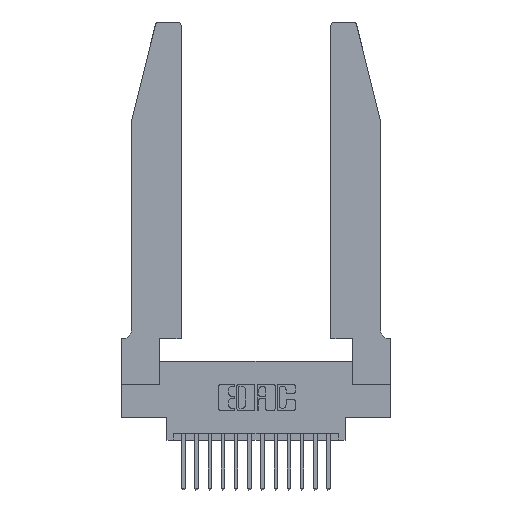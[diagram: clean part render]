
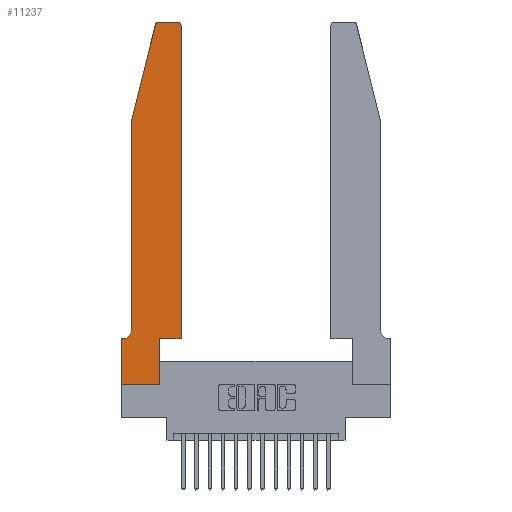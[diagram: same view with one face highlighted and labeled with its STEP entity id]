
A CAD part, top view. The second image highlights one B-rep face of the part: STEP entity #11237.
In plain terms, the highlighted planar face has unit normal (0, 0, 1).
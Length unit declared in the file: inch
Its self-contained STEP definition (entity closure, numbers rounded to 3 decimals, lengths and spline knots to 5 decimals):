
#123 = EDGE_CURVE ( 'NONE', #6997, #11160, #590, .T. ) ;
#590 = LINE ( 'NONE', #8348, #17667 ) ;
#595 = VECTOR ( 'NONE', #2272, 39.37008 ) ;
#698 = CARTESIAN_POINT ( 'NONE',  ( 0.2865, 0.35, 0.37 ) ) ;
#736 = ORIENTED_EDGE ( 'NONE', *, *, #9424, .T. ) ;
#827 = FACE_OUTER_BOUND ( 'NONE', #8961, .T. ) ;
#870 = LINE ( 'NONE', #10296, #5294 ) ;
#1381 = CARTESIAN_POINT ( 'NONE',  ( 0.2865, 0.35, 0.37 ) ) ;
#1463 = CARTESIAN_POINT ( 'NONE',  ( 0., 0., 0.37 ) ) ;
#1509 = CARTESIAN_POINT ( 'NONE',  ( 0., 0.35, 0.37 ) ) ;
#1594 = VERTEX_POINT ( 'NONE', #3056 ) ;
#1901 = CARTESIAN_POINT ( 'NONE',  ( 0.0755, 0.42, 0.37 ) ) ;
#1957 = ORIENTED_EDGE ( 'NONE', *, *, #18181, .T. ) ;
#2272 = DIRECTION ( 'NONE',  ( 1., 0., 0. ) ) ;
#2346 = EDGE_CURVE ( 'NONE', #17652, #11881, #870, .T. ) ;
#2435 = DIRECTION ( 'NONE',  ( 0., 0., 1. ) ) ;
#2855 = CARTESIAN_POINT ( 'NONE',  ( 0.25487, 2.72718, 0.37 ) ) ;
#2873 = ORIENTED_EDGE ( 'NONE', *, *, #4333, .T. ) ;
#2969 = ORIENTED_EDGE ( 'NONE', *, *, #4697, .T. ) ;
#3056 = CARTESIAN_POINT ( 'NONE',  ( 0.0755, 2., 0.37 ) ) ;
#3243 = CARTESIAN_POINT ( 'NONE',  ( 0.0755, 2., 0.37 ) ) ;
#3302 = LINE ( 'NONE', #13647, #17789 ) ;
#3532 = VERTEX_POINT ( 'NONE', #17469 ) ;
#4275 = CARTESIAN_POINT ( 'NONE',  ( 0.0755, 0.35, 0.37 ) ) ;
#4320 = DIRECTION ( 'NONE',  ( 1., 0., 0. ) ) ;
#4333 = EDGE_CURVE ( 'NONE', #5399, #3532, #4551, .T. ) ;
#4551 = LINE ( 'NONE', #9466, #595 ) ;
#4697 = EDGE_CURVE ( 'NONE', #1594, #5414, #14672, .T. ) ;
#5294 = VECTOR ( 'NONE', #10854, 39.37008 ) ;
#5344 = ORIENTED_EDGE ( 'NONE', *, *, #13227, .T. ) ;
#5399 = VERTEX_POINT ( 'NONE', #11874 ) ;
#5414 = VERTEX_POINT ( 'NONE', #1901 ) ;
#5489 = CARTESIAN_POINT ( 'NONE',  ( 0.284, 2.75, 0.37 ) ) ;
#6190 = DIRECTION ( 'NONE',  ( 0., -1., 0. ) ) ;
#6212 = EDGE_CURVE ( 'NONE', #11881, #6997, #9613, .T. ) ;
#6568 = DIRECTION ( 'NONE',  ( 0., 1., 0. ) ) ;
#6668 = ORIENTED_EDGE ( 'NONE', *, *, #6212, .T. ) ;
#6692 = VECTOR ( 'NONE', #8637, 39.37008 ) ;
#6775 = EDGE_CURVE ( 'NONE', #3532, #16432, #8300, .T. ) ;
#6997 = VERTEX_POINT ( 'NONE', #16781 ) ;
#7239 = CARTESIAN_POINT ( 'NONE',  ( 0.4505, 0.35, 0.37 ) ) ;
#7266 = VERTEX_POINT ( 'NONE', #8049 ) ;
#7330 = DIRECTION ( 'NONE',  ( -1., 0., 0. ) ) ;
#7344 = LINE ( 'NONE', #7239, #9823 ) ;
#7353 = AXIS2_PLACEMENT_3D ( 'NONE', #7497, #17211, #8926 ) ;
#7425 = ORIENTED_EDGE ( 'NONE', *, *, #2346, .T. ) ;
#7467 = ORIENTED_EDGE ( 'NONE', *, *, #123, .T. ) ;
#7497 = CARTESIAN_POINT ( 'NONE',  ( 0.284, 2.72, 0.37 ) ) ;
#7501 = ORIENTED_EDGE ( 'NONE', *, *, #6775, .T. ) ;
#7906 = DIRECTION ( 'NONE',  ( 0., 0., -1. ) ) ;
#8049 = CARTESIAN_POINT ( 'NONE',  ( 0.0055, 0.35, 0.37 ) ) ;
#8300 = LINE ( 'NONE', #698, #16101 ) ;
#8348 = CARTESIAN_POINT ( 'NONE',  ( 0.2605, 2.75, 0.37 ) ) ;
#8485 = DIRECTION ( 'NONE',  ( 0., 0., 1. ) ) ;
#8622 = AXIS2_PLACEMENT_3D ( 'NONE', #11003, #2435, #12408 ) ;
#8637 = DIRECTION ( 'NONE',  ( -1., 0., 0. ) ) ;
#8710 = EDGE_CURVE ( 'NONE', #7266, #10005, #10415, .T. ) ;
#8803 = DIRECTION ( 'NONE',  ( 0., -1., 0. ) ) ;
#8926 = DIRECTION ( 'NONE',  ( 1., 0., 0. ) ) ;
#8961 = EDGE_LOOP ( 'NONE', ( #7467, #11362, #18249, #2969, #1957, #15100, #5344, #2873, #7501, #736, #7425, #6668 ) ) ;
#9424 = EDGE_CURVE ( 'NONE', #16432, #17652, #7344, .T. ) ;
#9466 = CARTESIAN_POINT ( 'NONE',  ( 0., 0., 0.37 ) ) ;
#9613 = CIRCLE ( 'NONE', #8622, 0.03 ) ;
#9806 = PLANE ( 'NONE',  #17016 ) ;
#9823 = VECTOR ( 'NONE', #4320, 39.37008 ) ;
#9967 = CIRCLE ( 'NONE', #17928, 0.07 ) ;
#10005 = VERTEX_POINT ( 'NONE', #1509 ) ;
#10115 = VECTOR ( 'NONE', #6190, 39.37008 ) ;
#10296 = CARTESIAN_POINT ( 'NONE',  ( 0.4505, 0.35, 0.37 ) ) ;
#10415 = LINE ( 'NONE', #4275, #6692 ) ;
#10854 = DIRECTION ( 'NONE',  ( 0., 1., 0. ) ) ;
#11003 = CARTESIAN_POINT ( 'NONE',  ( 0.4205, 2.72, 0.37 ) ) ;
#11160 = VERTEX_POINT ( 'NONE', #5489 ) ;
#11237 = ADVANCED_FACE ( 'NONE', ( #827 ), #9806, .T. ) ;
#11362 = ORIENTED_EDGE ( 'NONE', *, *, #15876, .T. ) ;
#11874 = CARTESIAN_POINT ( 'NONE',  ( 0., 0., 0.37 ) ) ;
#11881 = VERTEX_POINT ( 'NONE', #16748 ) ;
#12408 = DIRECTION ( 'NONE',  ( 1., 0., 0. ) ) ;
#13227 = EDGE_CURVE ( 'NONE', #10005, #5399, #17639, .T. ) ;
#13647 = CARTESIAN_POINT ( 'NONE',  ( 0.0755, 2., 0.37 ) ) ;
#13977 = VECTOR ( 'NONE', #8803, 39.37008 ) ;
#14672 = LINE ( 'NONE', #3243, #10115 ) ;
#15063 = DIRECTION ( 'NONE',  ( -0.239, -0.971, 0. ) ) ;
#15100 = ORIENTED_EDGE ( 'NONE', *, *, #8710, .T. ) ;
#15824 = VERTEX_POINT ( 'NONE', #2855 ) ;
#15876 = EDGE_CURVE ( 'NONE', #11160, #15824, #16113, .T. ) ;
#16101 = VECTOR ( 'NONE', #6568, 39.37008 ) ;
#16113 = CIRCLE ( 'NONE', #7353, 0.03 ) ;
#16211 = CARTESIAN_POINT ( 'NONE',  ( 0.0055, 0.42, 0.37 ) ) ;
#16432 = VERTEX_POINT ( 'NONE', #1381 ) ;
#16686 = EDGE_CURVE ( 'NONE', #15824, #1594, #3302, .T. ) ;
#16748 = CARTESIAN_POINT ( 'NONE',  ( 0.4505, 2.72, 0.37 ) ) ;
#16773 = CARTESIAN_POINT ( 'NONE',  ( 0., 0.35, 0.37 ) ) ;
#16781 = CARTESIAN_POINT ( 'NONE',  ( 0.4205, 2.75, 0.37 ) ) ;
#17016 = AXIS2_PLACEMENT_3D ( 'NONE', #16773, #8485, #18147 ) ;
#17207 = CARTESIAN_POINT ( 'NONE',  ( 0.4505, 0.35, 0.37 ) ) ;
#17211 = DIRECTION ( 'NONE',  ( 0., 0., 1. ) ) ;
#17469 = CARTESIAN_POINT ( 'NONE',  ( 0.2865, 0., 0.37 ) ) ;
#17580 = DIRECTION ( 'NONE',  ( -1., 0., 0. ) ) ;
#17639 = LINE ( 'NONE', #1463, #13977 ) ;
#17652 = VERTEX_POINT ( 'NONE', #17207 ) ;
#17667 = VECTOR ( 'NONE', #7330, 39.37008 ) ;
#17789 = VECTOR ( 'NONE', #15063, 39.37008 ) ;
#17928 = AXIS2_PLACEMENT_3D ( 'NONE', #16211, #7906, #17580 ) ;
#18147 = DIRECTION ( 'NONE',  ( 1., 0., 0. ) ) ;
#18181 = EDGE_CURVE ( 'NONE', #5414, #7266, #9967, .T. ) ;
#18249 = ORIENTED_EDGE ( 'NONE', *, *, #16686, .T. ) ;
